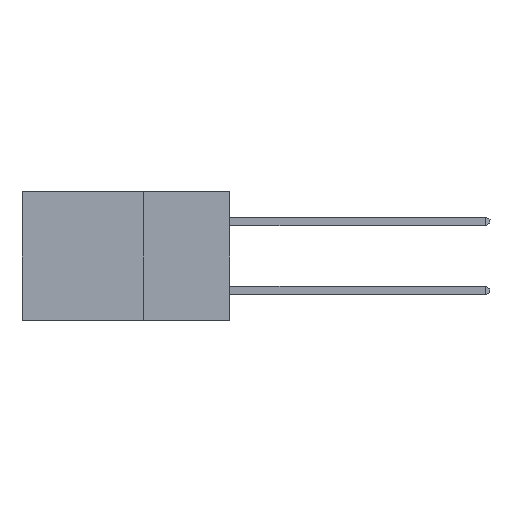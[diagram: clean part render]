
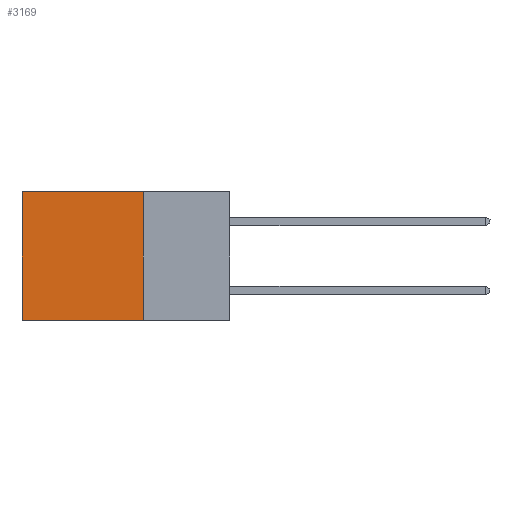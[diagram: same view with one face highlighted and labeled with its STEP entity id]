
A CAD part, left-side view. The second image highlights one B-rep face of the part: STEP entity #3169.
In plain terms, the highlighted planar face has unit normal (-1, 0, 0).
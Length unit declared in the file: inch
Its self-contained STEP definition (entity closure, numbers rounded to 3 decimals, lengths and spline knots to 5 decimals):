
#589 = VECTOR ( 'NONE', #6063, 39.37008 ) ;
#680 = LINE ( 'NONE', #5735, #1547 ) ;
#739 = PLANE ( 'NONE',  #3077 ) ;
#1063 = CARTESIAN_POINT ( 'NONE',  ( 0.2615, 0.25, -0.37 ) ) ;
#1547 = VECTOR ( 'NONE', #4151, 39.37008 ) ;
#1676 = VERTEX_POINT ( 'NONE', #3110 ) ;
#2772 = LINE ( 'NONE', #4513, #2888 ) ;
#2888 = VECTOR ( 'NONE', #3378, 39.37008 ) ;
#3077 = AXIS2_PLACEMENT_3D ( 'NONE', #6637, #8477, #6693 ) ;
#3110 = CARTESIAN_POINT ( 'NONE',  ( 0.2615, 0.6, 0. ) ) ;
#3169 = ADVANCED_FACE ( 'NONE', ( #6804 ), #739, .F. ) ;
#3378 = DIRECTION ( 'NONE',  ( 0., 0., -1. ) ) ;
#3783 = EDGE_CURVE ( 'NONE', #6833, #4094, #9595, .T. ) ;
#3942 = LINE ( 'NONE', #8154, #5069 ) ;
#4051 = DIRECTION ( 'NONE',  ( 0., 1., 0. ) ) ;
#4094 = VERTEX_POINT ( 'NONE', #5407 ) ;
#4095 = ORIENTED_EDGE ( 'NONE', *, *, #3783, .F. ) ;
#4151 = DIRECTION ( 'NONE',  ( 0., 1., 0. ) ) ;
#4360 = EDGE_CURVE ( 'NONE', #6833, #1676, #3942, .T. ) ;
#4513 = CARTESIAN_POINT ( 'NONE',  ( 0.2615, 0.6, -0.37 ) ) ;
#5069 = VECTOR ( 'NONE', #4051, 39.37008 ) ;
#5407 = CARTESIAN_POINT ( 'NONE',  ( 0.2615, 0.25, -0.37 ) ) ;
#5735 = CARTESIAN_POINT ( 'NONE',  ( 0.2615, 0.25, -0.37 ) ) ;
#6063 = DIRECTION ( 'NONE',  ( 0., 0., -1. ) ) ;
#6106 = CARTESIAN_POINT ( 'NONE',  ( 0.2615, 0.25, 0. ) ) ;
#6211 = VERTEX_POINT ( 'NONE', #7627 ) ;
#6637 = CARTESIAN_POINT ( 'NONE',  ( 0.2615, 0.25, -0.37 ) ) ;
#6693 = DIRECTION ( 'NONE',  ( 0., 0., -1. ) ) ;
#6804 = FACE_OUTER_BOUND ( 'NONE', #10899, .T. ) ;
#6833 = VERTEX_POINT ( 'NONE', #6106 ) ;
#7068 = ORIENTED_EDGE ( 'NONE', *, *, #10062, .F. ) ;
#7627 = CARTESIAN_POINT ( 'NONE',  ( 0.2615, 0.6, -0.37 ) ) ;
#8154 = CARTESIAN_POINT ( 'NONE',  ( 0.2615, 0.25, 0. ) ) ;
#8477 = DIRECTION ( 'NONE',  ( 1., 0., 0. ) ) ;
#8906 = ORIENTED_EDGE ( 'NONE', *, *, #4360, .T. ) ;
#9595 = LINE ( 'NONE', #1063, #589 ) ;
#10062 = EDGE_CURVE ( 'NONE', #4094, #6211, #680, .T. ) ;
#10423 = ORIENTED_EDGE ( 'NONE', *, *, #11016, .T. ) ;
#10899 = EDGE_LOOP ( 'NONE', ( #10423, #7068, #4095, #8906 ) ) ;
#11016 = EDGE_CURVE ( 'NONE', #1676, #6211, #2772, .T. ) ;
